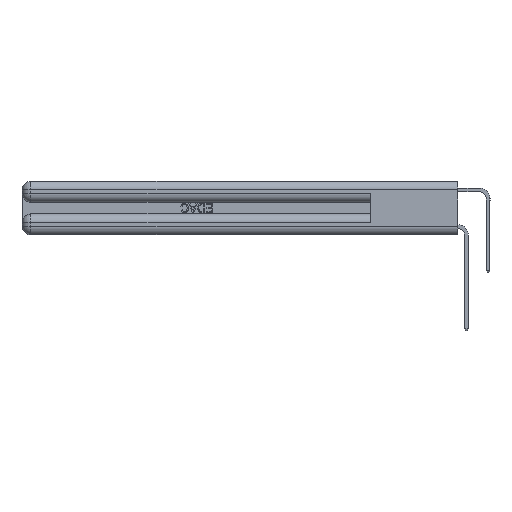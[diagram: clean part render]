
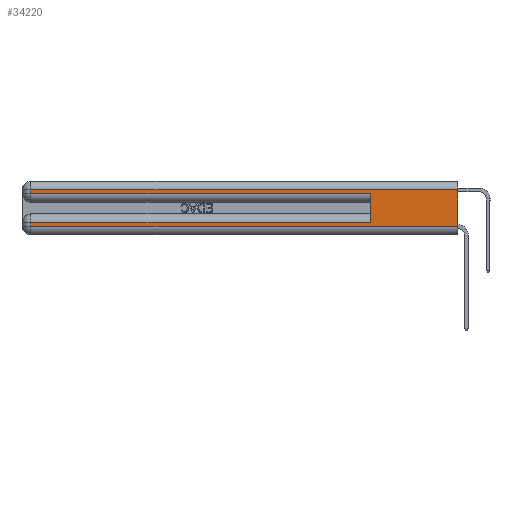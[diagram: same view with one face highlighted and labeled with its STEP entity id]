
A CAD part, left-side view. The second image highlights one B-rep face of the part: STEP entity #34220.
In plain terms, the highlighted planar face has unit normal (-1, 0, 0).
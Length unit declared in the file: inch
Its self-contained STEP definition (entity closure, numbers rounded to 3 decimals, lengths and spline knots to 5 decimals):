
#152 = VECTOR ( 'NONE', #22169, 39.37008 ) ;
#758 = VERTEX_POINT ( 'NONE', #14709 ) ;
#1872 = CARTESIAN_POINT ( 'NONE',  ( 0., 2.94, 0.37 ) ) ;
#2886 = CARTESIAN_POINT ( 'NONE',  ( 0., 0., 0.06 ) ) ;
#3244 = PLANE ( 'NONE',  #22442 ) ;
#3257 = CARTESIAN_POINT ( 'NONE',  ( 0., 0., 0.31 ) ) ;
#5236 = VECTOR ( 'NONE', #19887, 39.37008 ) ;
#6678 = ORIENTED_EDGE ( 'NONE', *, *, #19155, .T. ) ;
#7527 = EDGE_CURVE ( 'NONE', #17745, #28227, #29620, .T. ) ;
#8971 = VECTOR ( 'NONE', #16377, 39.37008 ) ;
#9110 = EDGE_CURVE ( 'NONE', #36154, #21919, #15571, .T. ) ;
#9361 = ORIENTED_EDGE ( 'NONE', *, *, #7527, .T. ) ;
#9551 = VECTOR ( 'NONE', #29899, 39.37008 ) ;
#9612 = DIRECTION ( 'NONE',  ( 0., 0., -1. ) ) ;
#10498 = ORIENTED_EDGE ( 'NONE', *, *, #21893, .F. ) ;
#10605 = ORIENTED_EDGE ( 'NONE', *, *, #18250, .T. ) ;
#10766 = VECTOR ( 'NONE', #27111, 39.37008 ) ;
#10914 = DIRECTION ( 'NONE',  ( 0., 0., -1. ) ) ;
#11367 = VERTEX_POINT ( 'NONE', #36596 ) ;
#11378 = DIRECTION ( 'NONE',  ( 0., 0., -1. ) ) ;
#11570 = CARTESIAN_POINT ( 'NONE',  ( 0., 2.94, 0.085 ) ) ;
#12116 = FACE_OUTER_BOUND ( 'NONE', #19516, .T. ) ;
#13129 = LINE ( 'NONE', #24868, #152 ) ;
#14335 = VECTOR ( 'NONE', #11378, 39.37008 ) ;
#14709 = CARTESIAN_POINT ( 'NONE',  ( 0., 2.94, 0.06 ) ) ;
#14919 = EDGE_CURVE ( 'NONE', #758, #26266, #16756, .T. ) ;
#15571 = LINE ( 'NONE', #27681, #10766 ) ;
#16095 = VECTOR ( 'NONE', #26756, 39.37008 ) ;
#16377 = DIRECTION ( 'NONE',  ( 0., -1., 0. ) ) ;
#16756 = LINE ( 'NONE', #19066, #8971 ) ;
#17745 = VERTEX_POINT ( 'NONE', #19815 ) ;
#18250 = EDGE_CURVE ( 'NONE', #28227, #20642, #37242, .T. ) ;
#19066 = CARTESIAN_POINT ( 'NONE',  ( 0., 0., 0.06 ) ) ;
#19155 = EDGE_CURVE ( 'NONE', #21919, #758, #13129, .T. ) ;
#19516 = EDGE_LOOP ( 'NONE', ( #10498, #9361, #10605, #30682, #21096, #19943, #6678, #33197 ) ) ;
#19815 = CARTESIAN_POINT ( 'NONE',  ( 0., 0., 0.31 ) ) ;
#19887 = DIRECTION ( 'NONE',  ( 0., -1., 0. ) ) ;
#19943 = ORIENTED_EDGE ( 'NONE', *, *, #9110, .T. ) ;
#20642 = VERTEX_POINT ( 'NONE', #29830 ) ;
#21096 = ORIENTED_EDGE ( 'NONE', *, *, #24707, .F. ) ;
#21893 = EDGE_CURVE ( 'NONE', #17745, #26266, #26202, .T. ) ;
#21919 = VERTEX_POINT ( 'NONE', #11570 ) ;
#22169 = DIRECTION ( 'NONE',  ( 0., 0., -1. ) ) ;
#22442 = AXIS2_PLACEMENT_3D ( 'NONE', #26365, #35937, #9612 ) ;
#22947 = CARTESIAN_POINT ( 'NONE',  ( 0., 0., 0.285 ) ) ;
#24707 = EDGE_CURVE ( 'NONE', #36154, #11367, #29500, .T. ) ;
#24868 = CARTESIAN_POINT ( 'NONE',  ( 0., 2.94, 0.37 ) ) ;
#26202 = LINE ( 'NONE', #32139, #14335 ) ;
#26266 = VERTEX_POINT ( 'NONE', #2886 ) ;
#26365 = CARTESIAN_POINT ( 'NONE',  ( 0., 0., 0.37 ) ) ;
#26756 = DIRECTION ( 'NONE',  ( 0., 1., 0. ) ) ;
#27020 = CARTESIAN_POINT ( 'NONE',  ( 0., 0.6, 0.145 ) ) ;
#27111 = DIRECTION ( 'NONE',  ( 0., 1., 0. ) ) ;
#27681 = CARTESIAN_POINT ( 'NONE',  ( 0., 0., 0.085 ) ) ;
#28227 = VERTEX_POINT ( 'NONE', #34964 ) ;
#28413 = CARTESIAN_POINT ( 'NONE',  ( 0., 0.6, 0.085 ) ) ;
#28540 = LINE ( 'NONE', #22947, #5236 ) ;
#29500 = LINE ( 'NONE', #27020, #9551 ) ;
#29620 = LINE ( 'NONE', #3257, #16095 ) ;
#29830 = CARTESIAN_POINT ( 'NONE',  ( 0., 2.94, 0.285 ) ) ;
#29899 = DIRECTION ( 'NONE',  ( 0., 0., 1. ) ) ;
#30682 = ORIENTED_EDGE ( 'NONE', *, *, #33680, .T. ) ;
#31450 = VECTOR ( 'NONE', #10914, 39.37008 ) ;
#32139 = CARTESIAN_POINT ( 'NONE',  ( 0., 0., 0.37 ) ) ;
#33197 = ORIENTED_EDGE ( 'NONE', *, *, #14919, .T. ) ;
#33680 = EDGE_CURVE ( 'NONE', #20642, #11367, #28540, .T. ) ;
#34220 = ADVANCED_FACE ( 'NONE', ( #12116 ), #3244, .F. ) ;
#34964 = CARTESIAN_POINT ( 'NONE',  ( 0., 2.94, 0.31 ) ) ;
#35937 = DIRECTION ( 'NONE',  ( 1., 0., 0. ) ) ;
#36154 = VERTEX_POINT ( 'NONE', #28413 ) ;
#36596 = CARTESIAN_POINT ( 'NONE',  ( 0., 0.6, 0.285 ) ) ;
#37242 = LINE ( 'NONE', #1872, #31450 ) ;
